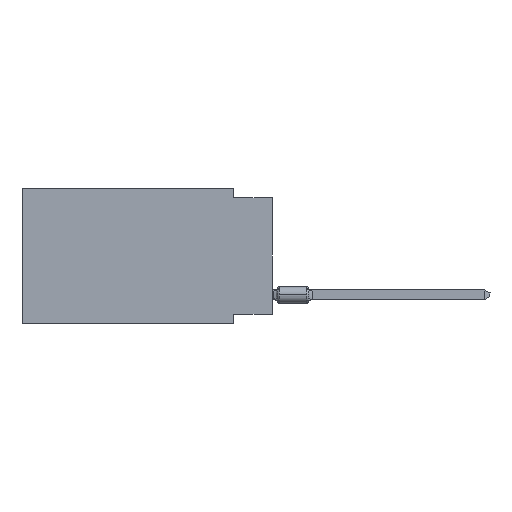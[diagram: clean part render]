
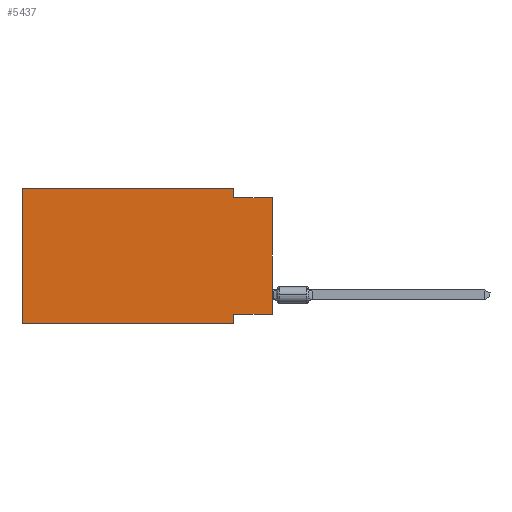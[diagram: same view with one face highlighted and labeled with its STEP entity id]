
A CAD part, left-side view. The second image highlights one B-rep face of the part: STEP entity #5437.
In plain terms, the highlighted planar face has unit normal (-1, 0, 0).
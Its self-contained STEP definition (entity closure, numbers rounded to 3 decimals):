
#3134 = EDGE_CURVE ( 'NONE', #94742, #45411, #49579, .T. ) ;
#5437 = ADVANCED_FACE ( 'NONE', ( #43769 ), #73071, .F. ) ;
#7449 = CARTESIAN_POINT ( 'NONE',  ( 0., 2.54, 0. ) ) ;
#8121 = CARTESIAN_POINT ( 'NONE',  ( 0., 2.54, -0.635 ) ) ;
#8335 = CARTESIAN_POINT ( 'NONE',  ( 0., 16.383, 0. ) ) ;
#9611 = ORIENTED_EDGE ( 'NONE', *, *, #12864, .F. ) ;
#10259 = VECTOR ( 'NONE', #52734, 1000. ) ;
#11348 = VERTEX_POINT ( 'NONE', #72964 ) ;
#11703 = CARTESIAN_POINT ( 'NONE',  ( 0., 0., -8.255 ) ) ;
#12137 = ORIENTED_EDGE ( 'NONE', *, *, #51003, .F. ) ;
#12864 = EDGE_CURVE ( 'NONE', #66018, #28187, #31880, .T. ) ;
#18021 = VECTOR ( 'NONE', #46072, 1000. ) ;
#23313 = ORIENTED_EDGE ( 'NONE', *, *, #57022, .F. ) ;
#27989 = LINE ( 'NONE', #7449, #29623 ) ;
#28004 = VECTOR ( 'NONE', #70839, 1000. ) ;
#28158 = DIRECTION ( 'NONE',  ( 1., 0., 0. ) ) ;
#28187 = VERTEX_POINT ( 'NONE', #54368 ) ;
#28968 = DIRECTION ( 'NONE',  ( 0., 0., -1. ) ) ;
#29623 = VECTOR ( 'NONE', #28968, 1000. ) ;
#29804 = CARTESIAN_POINT ( 'NONE',  ( 0., 2.54, -8.89 ) ) ;
#30107 = CARTESIAN_POINT ( 'NONE',  ( 0., 16.383, 0. ) ) ;
#30523 = ORIENTED_EDGE ( 'NONE', *, *, #63036, .T. ) ;
#31880 = LINE ( 'NONE', #61646, #35867 ) ;
#32018 = CARTESIAN_POINT ( 'NONE',  ( 0., 16.383, 0. ) ) ;
#32219 = ORIENTED_EDGE ( 'NONE', *, *, #3134, .F. ) ;
#32711 = CARTESIAN_POINT ( 'NONE',  ( 0., 2.54, 0. ) ) ;
#34936 = VERTEX_POINT ( 'NONE', #32711 ) ;
#35867 = VECTOR ( 'NONE', #91422, 1000. ) ;
#36817 = VERTEX_POINT ( 'NONE', #88978 ) ;
#37182 = EDGE_CURVE ( 'NONE', #28187, #11348, #51283, .T. ) ;
#37787 = CARTESIAN_POINT ( 'NONE',  ( 0., 0., 0. ) ) ;
#38514 = EDGE_CURVE ( 'NONE', #45411, #34936, #75237, .T. ) ;
#43425 = VECTOR ( 'NONE', #68405, 1000. ) ;
#43769 = FACE_OUTER_BOUND ( 'NONE', #78728, .T. ) ;
#45411 = VERTEX_POINT ( 'NONE', #32018 ) ;
#45453 = LINE ( 'NONE', #75219, #94256 ) ;
#46072 = DIRECTION ( 'NONE',  ( 0., 0., 1. ) ) ;
#49579 = LINE ( 'NONE', #94962, #87253 ) ;
#51003 = EDGE_CURVE ( 'NONE', #59516, #36817, #45453, .T. ) ;
#51283 = LINE ( 'NONE', #29804, #10259 ) ;
#52734 = DIRECTION ( 'NONE',  ( 0., 0., -1. ) ) ;
#54368 = CARTESIAN_POINT ( 'NONE',  ( 0., 2.54, -8.255 ) ) ;
#56191 = CARTESIAN_POINT ( 'NONE',  ( 0., 16.383, -8.89 ) ) ;
#57022 = EDGE_CURVE ( 'NONE', #34936, #59516, #27989, .T. ) ;
#59516 = VERTEX_POINT ( 'NONE', #8121 ) ;
#59695 = AXIS2_PLACEMENT_3D ( 'NONE', #30107, #28158, #89171 ) ;
#61646 = CARTESIAN_POINT ( 'NONE',  ( 0., 0., -8.255 ) ) ;
#63036 = EDGE_CURVE ( 'NONE', #66018, #36817, #76792, .T. ) ;
#66018 = VERTEX_POINT ( 'NONE', #11703 ) ;
#67574 = ORIENTED_EDGE ( 'NONE', *, *, #37182, .F. ) ;
#68405 = DIRECTION ( 'NONE',  ( 0., -1., 0. ) ) ;
#70762 = DIRECTION ( 'NONE',  ( 0., -1., 0. ) ) ;
#70839 = DIRECTION ( 'NONE',  ( 0., -1., 0. ) ) ;
#72293 = LINE ( 'NONE', #56191, #28004 ) ;
#72964 = CARTESIAN_POINT ( 'NONE',  ( 0., 2.54, -8.89 ) ) ;
#73071 = PLANE ( 'NONE',  #59695 ) ;
#75219 = CARTESIAN_POINT ( 'NONE',  ( 0., 0., -0.635 ) ) ;
#75237 = LINE ( 'NONE', #8335, #43425 ) ;
#76792 = LINE ( 'NONE', #37787, #18021 ) ;
#78728 = EDGE_LOOP ( 'NONE', ( #30523, #12137, #23313, #94770, #32219, #87101, #67574, #9611 ) ) ;
#79332 = DIRECTION ( 'NONE',  ( 0., 0., 1. ) ) ;
#87101 = ORIENTED_EDGE ( 'NONE', *, *, #88192, .T. ) ;
#87253 = VECTOR ( 'NONE', #79332, 1000. ) ;
#88192 = EDGE_CURVE ( 'NONE', #94742, #11348, #72293, .T. ) ;
#88978 = CARTESIAN_POINT ( 'NONE',  ( 0., 0., -0.635 ) ) ;
#89171 = DIRECTION ( 'NONE',  ( 0., 0., -1. ) ) ;
#91422 = DIRECTION ( 'NONE',  ( 0., 1., 0. ) ) ;
#91538 = CARTESIAN_POINT ( 'NONE',  ( 0., 16.383, -8.89 ) ) ;
#94256 = VECTOR ( 'NONE', #70762, 1000. ) ;
#94742 = VERTEX_POINT ( 'NONE', #91538 ) ;
#94770 = ORIENTED_EDGE ( 'NONE', *, *, #38514, .F. ) ;
#94962 = CARTESIAN_POINT ( 'NONE',  ( 0., 16.383, 0. ) ) ;
